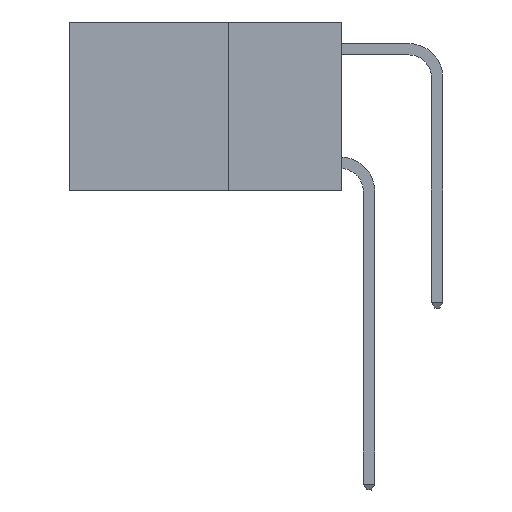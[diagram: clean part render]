
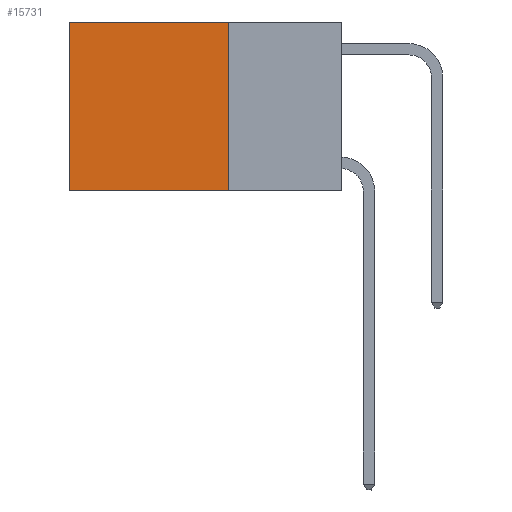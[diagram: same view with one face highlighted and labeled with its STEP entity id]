
A CAD part, left-side view. The second image highlights one B-rep face of the part: STEP entity #15731.
In plain terms, the highlighted planar face has unit normal (-1, 0, 0).
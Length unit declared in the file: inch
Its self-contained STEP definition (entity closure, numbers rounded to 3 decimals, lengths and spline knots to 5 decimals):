
#1566 = VERTEX_POINT ( 'NONE', #18119 ) ;
#1978 = LINE ( 'NONE', #4937, #6083 ) ;
#2486 = VERTEX_POINT ( 'NONE', #11907 ) ;
#2647 = VECTOR ( 'NONE', #10601, 39.37008 ) ;
#3287 = VERTEX_POINT ( 'NONE', #17387 ) ;
#3586 = PLANE ( 'NONE',  #19112 ) ;
#4937 = CARTESIAN_POINT ( 'NONE',  ( 0.2625, 0.25, 0. ) ) ;
#5140 = CARTESIAN_POINT ( 'NONE',  ( 0.2625, 0.25, 0. ) ) ;
#5790 = EDGE_CURVE ( 'NONE', #15726, #2486, #12186, .T. ) ;
#5950 = CARTESIAN_POINT ( 'NONE',  ( 0.2625, 0.6, 0. ) ) ;
#6083 = VECTOR ( 'NONE', #11124, 39.37008 ) ;
#6667 = DIRECTION ( 'NONE',  ( 0., 0., -1. ) ) ;
#6683 = EDGE_LOOP ( 'NONE', ( #13385, #17378, #8645, #14300 ) ) ;
#7631 = VECTOR ( 'NONE', #12687, 39.37008 ) ;
#8066 = CARTESIAN_POINT ( 'NONE',  ( 0.2625, 0.25, 0. ) ) ;
#8166 = CARTESIAN_POINT ( 'NONE',  ( 0.2625, 0.25, 0. ) ) ;
#8645 = ORIENTED_EDGE ( 'NONE', *, *, #17517, .F. ) ;
#9739 = LINE ( 'NONE', #16784, #17399 ) ;
#10601 = DIRECTION ( 'NONE',  ( 0., 0., -1. ) ) ;
#11124 = DIRECTION ( 'NONE',  ( 0., 0., -1. ) ) ;
#11907 = CARTESIAN_POINT ( 'NONE',  ( 0.2625, 0.6, 0. ) ) ;
#12186 = LINE ( 'NONE', #8066, #7631 ) ;
#12687 = DIRECTION ( 'NONE',  ( 0., 1., 0. ) ) ;
#13385 = ORIENTED_EDGE ( 'NONE', *, *, #18636, .T. ) ;
#13765 = DIRECTION ( 'NONE',  ( 0., 1., 0. ) ) ;
#14300 = ORIENTED_EDGE ( 'NONE', *, *, #5790, .T. ) ;
#15726 = VERTEX_POINT ( 'NONE', #8166 ) ;
#15731 = ADVANCED_FACE ( 'NONE', ( #17908 ), #3586, .F. ) ;
#15885 = DIRECTION ( 'NONE',  ( 1., 0., 0. ) ) ;
#16688 = EDGE_CURVE ( 'NONE', #1566, #3287, #9739, .T. ) ;
#16784 = CARTESIAN_POINT ( 'NONE',  ( 0.2625, 0.25, -0.37 ) ) ;
#17378 = ORIENTED_EDGE ( 'NONE', *, *, #16688, .F. ) ;
#17387 = CARTESIAN_POINT ( 'NONE',  ( 0.2625, 0.6, -0.37 ) ) ;
#17399 = VECTOR ( 'NONE', #13765, 39.37008 ) ;
#17517 = EDGE_CURVE ( 'NONE', #15726, #1566, #1978, .T. ) ;
#17908 = FACE_OUTER_BOUND ( 'NONE', #6683, .T. ) ;
#18119 = CARTESIAN_POINT ( 'NONE',  ( 0.2625, 0.25, -0.37 ) ) ;
#18636 = EDGE_CURVE ( 'NONE', #2486, #3287, #19454, .T. ) ;
#19112 = AXIS2_PLACEMENT_3D ( 'NONE', #5140, #15885, #6667 ) ;
#19454 = LINE ( 'NONE', #5950, #2647 ) ;
